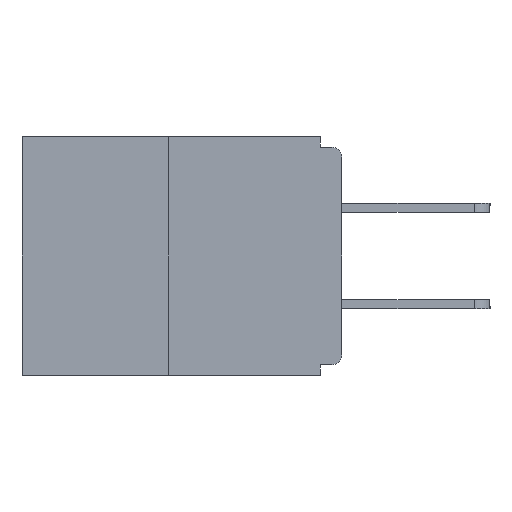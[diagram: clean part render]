
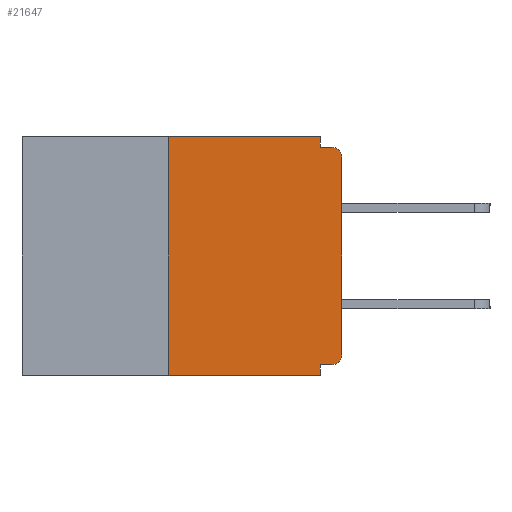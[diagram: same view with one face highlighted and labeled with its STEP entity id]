
A CAD part, left-side view. The second image highlights one B-rep face of the part: STEP entity #21647.
In plain terms, the highlighted planar face has unit normal (-1, 0, 0).
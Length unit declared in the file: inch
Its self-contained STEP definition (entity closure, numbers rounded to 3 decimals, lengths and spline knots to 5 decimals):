
#384 = CARTESIAN_POINT ( 'NONE',  ( 0., 0.46, 0. ) ) ;
#413 = EDGE_CURVE ( 'NONE', #15537, #14155, #15152, .T. ) ;
#801 = CARTESIAN_POINT ( 'NONE',  ( 0., 0.015, -0.03 ) ) ;
#943 = VECTOR ( 'NONE', #14865, 39.37008 ) ;
#1030 = DIRECTION ( 'NONE',  ( 0., -1., 0. ) ) ;
#1311 = DIRECTION ( 'NONE',  ( -1., 0., 0. ) ) ;
#1771 = CIRCLE ( 'NONE', #17382, 0.015 ) ;
#2068 = VERTEX_POINT ( 'NONE', #14411 ) ;
#2338 = LINE ( 'NONE', #15185, #17086 ) ;
#3103 = ORIENTED_EDGE ( 'NONE', *, *, #7235, .F. ) ;
#3263 = LINE ( 'NONE', #9708, #12949 ) ;
#3411 = CARTESIAN_POINT ( 'NONE',  ( 0., 0.031, -0.015 ) ) ;
#3996 = VERTEX_POINT ( 'NONE', #18203 ) ;
#4370 = VERTEX_POINT ( 'NONE', #5771 ) ;
#4576 = CARTESIAN_POINT ( 'NONE',  ( 0., 0.25, 0. ) ) ;
#4959 = CARTESIAN_POINT ( 'NONE',  ( 0., 0., -0.313 ) ) ;
#5003 = VERTEX_POINT ( 'NONE', #3411 ) ;
#5400 = VECTOR ( 'NONE', #11309, 39.37008 ) ;
#5587 = VECTOR ( 'NONE', #18491, 39.37008 ) ;
#5712 = VECTOR ( 'NONE', #15738, 39.37008 ) ;
#5771 = CARTESIAN_POINT ( 'NONE',  ( 0., 0.25, -0.343 ) ) ;
#5909 = DIRECTION ( 'NONE',  ( 0., 0., -1. ) ) ;
#6527 = ORIENTED_EDGE ( 'NONE', *, *, #23416, .T. ) ;
#6754 = CARTESIAN_POINT ( 'NONE',  ( 0., 0.015, -0.313 ) ) ;
#6758 = DIRECTION ( 'NONE',  ( 1., 0., 0. ) ) ;
#6937 = EDGE_CURVE ( 'NONE', #19503, #17486, #17237, .T. ) ;
#7047 = ORIENTED_EDGE ( 'NONE', *, *, #6937, .T. ) ;
#7235 = EDGE_CURVE ( 'NONE', #4370, #15537, #10490, .T. ) ;
#7854 = CARTESIAN_POINT ( 'NONE',  ( 0., 0.015, -0.015 ) ) ;
#8293 = VECTOR ( 'NONE', #16542, 39.37008 ) ;
#8475 = PLANE ( 'NONE',  #19206 ) ;
#8802 = CARTESIAN_POINT ( 'NONE',  ( 0., 0.46, 0. ) ) ;
#9436 = CARTESIAN_POINT ( 'NONE',  ( 0., 0.25, 0. ) ) ;
#9708 = CARTESIAN_POINT ( 'NONE',  ( 0., 0.031, 0. ) ) ;
#10255 = ORIENTED_EDGE ( 'NONE', *, *, #16783, .T. ) ;
#10490 = LINE ( 'NONE', #9436, #5587 ) ;
#10904 = EDGE_CURVE ( 'NONE', #19503, #19175, #20411, .T. ) ;
#11120 = CARTESIAN_POINT ( 'NONE',  ( 0., 0., 0. ) ) ;
#11188 = CARTESIAN_POINT ( 'NONE',  ( 0., 0.031, 0. ) ) ;
#11230 = CARTESIAN_POINT ( 'NONE',  ( 0., 0., -0.328 ) ) ;
#11309 = DIRECTION ( 'NONE',  ( 0., 1., 0. ) ) ;
#11794 = DIRECTION ( 'NONE',  ( 0., 0., -1. ) ) ;
#12154 = ORIENTED_EDGE ( 'NONE', *, *, #21320, .F. ) ;
#12818 = ORIENTED_EDGE ( 'NONE', *, *, #16708, .F. ) ;
#12949 = VECTOR ( 'NONE', #5909, 39.37008 ) ;
#13268 = DIRECTION ( 'NONE',  ( 0., 0., -1. ) ) ;
#13349 = CARTESIAN_POINT ( 'NONE',  ( 0., 0.031, -0.328 ) ) ;
#13812 = VECTOR ( 'NONE', #13268, 39.37008 ) ;
#14155 = VERTEX_POINT ( 'NONE', #11188 ) ;
#14308 = EDGE_LOOP ( 'NONE', ( #21006, #3103, #6527, #12154, #15184, #7047, #15881, #10255, #12818, #14887 ) ) ;
#14411 = CARTESIAN_POINT ( 'NONE',  ( 0., 0., -0.03 ) ) ;
#14865 = DIRECTION ( 'NONE',  ( 0., -1., 0. ) ) ;
#14887 = ORIENTED_EDGE ( 'NONE', *, *, #21348, .F. ) ;
#15152 = LINE ( 'NONE', #384, #943 ) ;
#15184 = ORIENTED_EDGE ( 'NONE', *, *, #10904, .F. ) ;
#15185 = CARTESIAN_POINT ( 'NONE',  ( 0., 0., -0.015 ) ) ;
#15230 = CARTESIAN_POINT ( 'NONE',  ( 0., 0.031, -0.343 ) ) ;
#15537 = VERTEX_POINT ( 'NONE', #4576 ) ;
#15738 = DIRECTION ( 'NONE',  ( 0., -1., 0. ) ) ;
#15881 = ORIENTED_EDGE ( 'NONE', *, *, #17818, .T. ) ;
#16323 = FACE_OUTER_BOUND ( 'NONE', #14308, .T. ) ;
#16542 = DIRECTION ( 'NONE',  ( 0., 0., 1. ) ) ;
#16708 = EDGE_CURVE ( 'NONE', #5003, #20691, #2338, .T. ) ;
#16783 = EDGE_CURVE ( 'NONE', #2068, #20691, #1771, .T. ) ;
#17086 = VECTOR ( 'NONE', #1030, 39.37008 ) ;
#17237 = CIRCLE ( 'NONE', #19730, 0.015 ) ;
#17382 = AXIS2_PLACEMENT_3D ( 'NONE', #801, #22590, #11794 ) ;
#17486 = VERTEX_POINT ( 'NONE', #4959 ) ;
#17818 = EDGE_CURVE ( 'NONE', #17486, #2068, #18481, .T. ) ;
#18203 = CARTESIAN_POINT ( 'NONE',  ( 0., 0.031, -0.343 ) ) ;
#18467 = LINE ( 'NONE', #20920, #5712 ) ;
#18481 = LINE ( 'NONE', #11120, #8293 ) ;
#18491 = DIRECTION ( 'NONE',  ( 0., 0., 1. ) ) ;
#19175 = VERTEX_POINT ( 'NONE', #13349 ) ;
#19206 = AXIS2_PLACEMENT_3D ( 'NONE', #8802, #6758, #21354 ) ;
#19503 = VERTEX_POINT ( 'NONE', #22466 ) ;
#19730 = AXIS2_PLACEMENT_3D ( 'NONE', #6754, #1311, #22950 ) ;
#20411 = LINE ( 'NONE', #11230, #5400 ) ;
#20691 = VERTEX_POINT ( 'NONE', #7854 ) ;
#20920 = CARTESIAN_POINT ( 'NONE',  ( 0., 0.46, -0.343 ) ) ;
#21006 = ORIENTED_EDGE ( 'NONE', *, *, #413, .F. ) ;
#21320 = EDGE_CURVE ( 'NONE', #19175, #3996, #22244, .T. ) ;
#21348 = EDGE_CURVE ( 'NONE', #14155, #5003, #3263, .T. ) ;
#21354 = DIRECTION ( 'NONE',  ( 0., 0., -1. ) ) ;
#21647 = ADVANCED_FACE ( 'NONE', ( #16323 ), #8475, .F. ) ;
#22244 = LINE ( 'NONE', #15230, #13812 ) ;
#22466 = CARTESIAN_POINT ( 'NONE',  ( 0., 0.015, -0.328 ) ) ;
#22590 = DIRECTION ( 'NONE',  ( -1., 0., 0. ) ) ;
#22950 = DIRECTION ( 'NONE',  ( 0., 0., -1. ) ) ;
#23416 = EDGE_CURVE ( 'NONE', #4370, #3996, #18467, .T. ) ;
